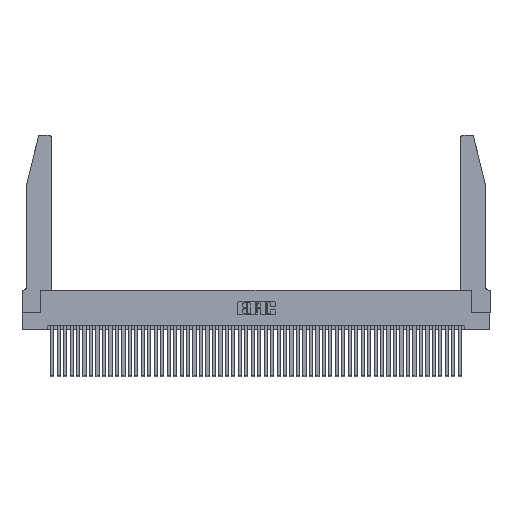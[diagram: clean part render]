
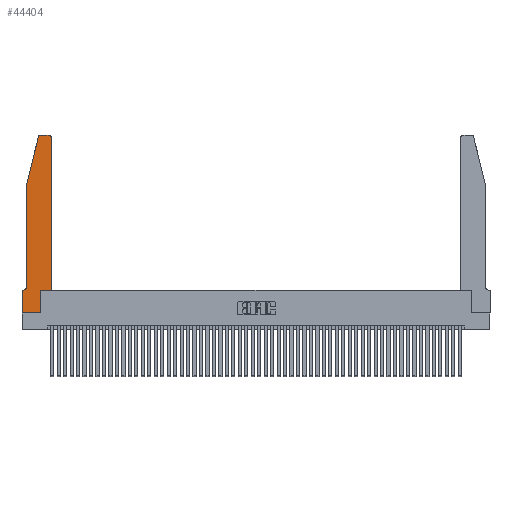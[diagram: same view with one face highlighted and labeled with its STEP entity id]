
A CAD part, top view. The second image highlights one B-rep face of the part: STEP entity #44404.
In plain terms, the highlighted planar face has unit normal (0, 0, 1).
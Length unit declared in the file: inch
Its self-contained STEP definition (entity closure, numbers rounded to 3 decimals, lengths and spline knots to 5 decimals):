
#961 = AXIS2_PLACEMENT_3D ( 'NONE', #7405, #23494, #42955 ) ;
#1908 = CARTESIAN_POINT ( 'NONE',  ( 0.2865, 0.35, 0.37 ) ) ;
#2795 = CARTESIAN_POINT ( 'NONE',  ( 0.284, 2.72, 0.37 ) ) ;
#3346 = DIRECTION ( 'NONE',  ( -1., 0., 0. ) ) ;
#3691 = CARTESIAN_POINT ( 'NONE',  ( 0.2605, 2.75, 0.37 ) ) ;
#3897 = VERTEX_POINT ( 'NONE', #40674 ) ;
#3907 = ORIENTED_EDGE ( 'NONE', *, *, #16751, .T. ) ;
#4078 = VERTEX_POINT ( 'NONE', #42038 ) ;
#4415 = CARTESIAN_POINT ( 'NONE',  ( 0., 0.35, 0.37 ) ) ;
#4630 = EDGE_CURVE ( 'NONE', #5008, #45765, #43010, .T. ) ;
#5008 = VERTEX_POINT ( 'NONE', #46655 ) ;
#5813 = AXIS2_PLACEMENT_3D ( 'NONE', #16808, #40829, #44649 ) ;
#6150 = EDGE_CURVE ( 'NONE', #16559, #36280, #51623, .T. ) ;
#6264 = CARTESIAN_POINT ( 'NONE',  ( 0.4505, 0.35, 0.37 ) ) ;
#6438 = DIRECTION ( 'NONE',  ( 0., 1., 0. ) ) ;
#7378 = CARTESIAN_POINT ( 'NONE',  ( 0.4205, 2.75, 0.37 ) ) ;
#7405 = CARTESIAN_POINT ( 'NONE',  ( 0.4205, 2.72, 0.37 ) ) ;
#10021 = CARTESIAN_POINT ( 'NONE',  ( 0.284, 2.75, 0.37 ) ) ;
#10176 = LINE ( 'NONE', #39535, #45863 ) ;
#10316 = VERTEX_POINT ( 'NONE', #23962 ) ;
#10477 = CARTESIAN_POINT ( 'NONE',  ( 0.2865, 0., 0.37 ) ) ;
#11906 = VECTOR ( 'NONE', #39880, 39.37008 ) ;
#11936 = VERTEX_POINT ( 'NONE', #10477 ) ;
#12141 = PLANE ( 'NONE',  #18140 ) ;
#12150 = EDGE_CURVE ( 'NONE', #4078, #27919, #12152, .T. ) ;
#12152 = LINE ( 'NONE', #47531, #27823 ) ;
#12608 = EDGE_CURVE ( 'NONE', #27985, #16559, #26500, .T. ) ;
#13232 = EDGE_CURVE ( 'NONE', #36280, #4078, #16432, .T. ) ;
#13732 = VERTEX_POINT ( 'NONE', #30222 ) ;
#14341 = LINE ( 'NONE', #25703, #39417 ) ;
#14941 = VECTOR ( 'NONE', #45268, 39.37008 ) ;
#15182 = EDGE_CURVE ( 'NONE', #27919, #13732, #18797, .T. ) ;
#15438 = CARTESIAN_POINT ( 'NONE',  ( 0.0755, 2., 0.37 ) ) ;
#15492 = ORIENTED_EDGE ( 'NONE', *, *, #12608, .T. ) ;
#15555 = DIRECTION ( 'NONE',  ( 1., 0., 0. ) ) ;
#15776 = CARTESIAN_POINT ( 'NONE',  ( 0.4505, 2.72, 0.37 ) ) ;
#15998 = ORIENTED_EDGE ( 'NONE', *, *, #45619, .T. ) ;
#16340 = DIRECTION ( 'NONE',  ( 0., 0., 1. ) ) ;
#16432 = CIRCLE ( 'NONE', #49968, 0.03 ) ;
#16559 = VERTEX_POINT ( 'NONE', #7378 ) ;
#16751 = EDGE_CURVE ( 'NONE', #13732, #5008, #18155, .T. ) ;
#16808 = CARTESIAN_POINT ( 'NONE',  ( 0.0055, 0.42, 0.37 ) ) ;
#16948 = DIRECTION ( 'NONE',  ( -1., 0., 0. ) ) ;
#17015 = VERTEX_POINT ( 'NONE', #6264 ) ;
#17459 = EDGE_CURVE ( 'NONE', #45765, #10316, #23067, .T. ) ;
#17863 = ORIENTED_EDGE ( 'NONE', *, *, #50755, .T. ) ;
#18140 = AXIS2_PLACEMENT_3D ( 'NONE', #4415, #16340, #20359 ) ;
#18155 = CIRCLE ( 'NONE', #5813, 0.07 ) ;
#18218 = DIRECTION ( 'NONE',  ( 0., 1., 0. ) ) ;
#18797 = LINE ( 'NONE', #23586, #11906 ) ;
#19459 = VECTOR ( 'NONE', #18218, 39.37008 ) ;
#20359 = DIRECTION ( 'NONE',  ( 1., 0., 0. ) ) ;
#21095 = VECTOR ( 'NONE', #16948, 39.37008 ) ;
#22399 = DIRECTION ( 'NONE',  ( 1., 0., 0. ) ) ;
#22916 = DIRECTION ( 'NONE',  ( 0., 0., 1. ) ) ;
#23067 = LINE ( 'NONE', #37395, #14941 ) ;
#23494 = DIRECTION ( 'NONE',  ( 0., 0., 1. ) ) ;
#23586 = CARTESIAN_POINT ( 'NONE',  ( 0.0755, 2., 0.37 ) ) ;
#23825 = LINE ( 'NONE', #42202, #19459 ) ;
#23930 = FACE_OUTER_BOUND ( 'NONE', #29568, .T. ) ;
#23962 = CARTESIAN_POINT ( 'NONE',  ( 0., 0., 0.37 ) ) ;
#24367 = EDGE_CURVE ( 'NONE', #17015, #27985, #23825, .T. ) ;
#25703 = CARTESIAN_POINT ( 'NONE',  ( 0., 0., 0.37 ) ) ;
#26500 = CIRCLE ( 'NONE', #961, 0.03 ) ;
#27823 = VECTOR ( 'NONE', #51562, 39.37008 ) ;
#27919 = VERTEX_POINT ( 'NONE', #15438 ) ;
#27985 = VERTEX_POINT ( 'NONE', #15776 ) ;
#29568 = EDGE_LOOP ( 'NONE', ( #35909, #50251, #39831, #30926, #3907, #50674, #40544, #17863, #15998, #43462, #41378, #15492 ) ) ;
#30222 = CARTESIAN_POINT ( 'NONE',  ( 0.0755, 0.42, 0.37 ) ) ;
#30926 = ORIENTED_EDGE ( 'NONE', *, *, #15182, .T. ) ;
#31336 = EDGE_CURVE ( 'NONE', #3897, #17015, #10176, .T. ) ;
#33419 = VECTOR ( 'NONE', #3346, 39.37008 ) ;
#35475 = CARTESIAN_POINT ( 'NONE',  ( 0., 0.35, 0.37 ) ) ;
#35909 = ORIENTED_EDGE ( 'NONE', *, *, #6150, .T. ) ;
#36280 = VERTEX_POINT ( 'NONE', #10021 ) ;
#37395 = CARTESIAN_POINT ( 'NONE',  ( 0., 0., 0.37 ) ) ;
#37424 = CARTESIAN_POINT ( 'NONE',  ( 0.0755, 0.35, 0.37 ) ) ;
#39417 = VECTOR ( 'NONE', #42341, 39.37008 ) ;
#39535 = CARTESIAN_POINT ( 'NONE',  ( 0.4505, 0.35, 0.37 ) ) ;
#39831 = ORIENTED_EDGE ( 'NONE', *, *, #12150, .T. ) ;
#39880 = DIRECTION ( 'NONE',  ( 0., -1., 0. ) ) ;
#40544 = ORIENTED_EDGE ( 'NONE', *, *, #17459, .T. ) ;
#40674 = CARTESIAN_POINT ( 'NONE',  ( 0.2865, 0.35, 0.37 ) ) ;
#40829 = DIRECTION ( 'NONE',  ( 0., 0., -1. ) ) ;
#41378 = ORIENTED_EDGE ( 'NONE', *, *, #24367, .T. ) ;
#42038 = CARTESIAN_POINT ( 'NONE',  ( 0.25487, 2.72718, 0.37 ) ) ;
#42202 = CARTESIAN_POINT ( 'NONE',  ( 0.4505, 0.35, 0.37 ) ) ;
#42341 = DIRECTION ( 'NONE',  ( 1., 0., 0. ) ) ;
#42630 = VECTOR ( 'NONE', #6438, 39.37008 ) ;
#42955 = DIRECTION ( 'NONE',  ( 1., 0., 0. ) ) ;
#43010 = LINE ( 'NONE', #37424, #21095 ) ;
#43462 = ORIENTED_EDGE ( 'NONE', *, *, #31336, .T. ) ;
#43886 = LINE ( 'NONE', #1908, #42630 ) ;
#44404 = ADVANCED_FACE ( 'NONE', ( #23930 ), #12141, .T. ) ;
#44649 = DIRECTION ( 'NONE',  ( -1., 0., 0. ) ) ;
#45268 = DIRECTION ( 'NONE',  ( 0., -1., 0. ) ) ;
#45619 = EDGE_CURVE ( 'NONE', #11936, #3897, #43886, .T. ) ;
#45765 = VERTEX_POINT ( 'NONE', #35475 ) ;
#45863 = VECTOR ( 'NONE', #15555, 39.37008 ) ;
#46655 = CARTESIAN_POINT ( 'NONE',  ( 0.0055, 0.35, 0.37 ) ) ;
#47531 = CARTESIAN_POINT ( 'NONE',  ( 0.0755, 2., 0.37 ) ) ;
#49968 = AXIS2_PLACEMENT_3D ( 'NONE', #2795, #22916, #22399 ) ;
#50251 = ORIENTED_EDGE ( 'NONE', *, *, #13232, .T. ) ;
#50674 = ORIENTED_EDGE ( 'NONE', *, *, #4630, .T. ) ;
#50755 = EDGE_CURVE ( 'NONE', #10316, #11936, #14341, .T. ) ;
#51562 = DIRECTION ( 'NONE',  ( -0.239, -0.971, 0. ) ) ;
#51623 = LINE ( 'NONE', #3691, #33419 ) ;
